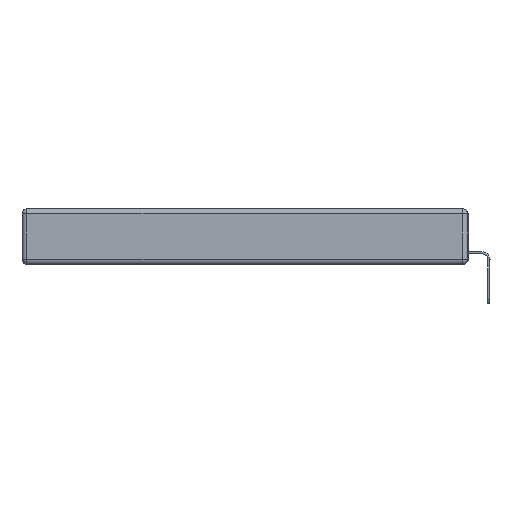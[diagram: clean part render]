
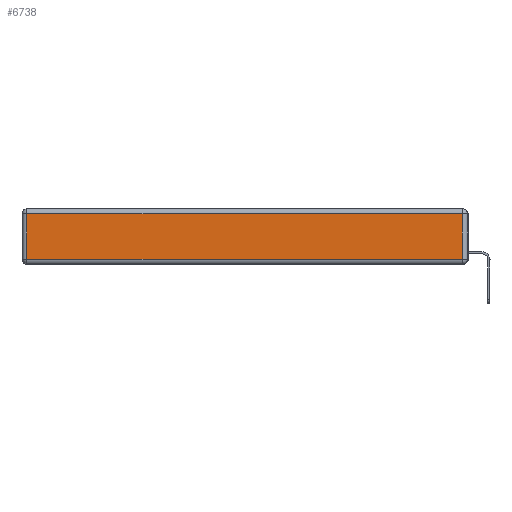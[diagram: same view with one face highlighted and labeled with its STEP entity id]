
A CAD part, left-side view. The second image highlights one B-rep face of the part: STEP entity #6738.
In plain terms, the highlighted planar face has unit normal (-1, 0, 0).
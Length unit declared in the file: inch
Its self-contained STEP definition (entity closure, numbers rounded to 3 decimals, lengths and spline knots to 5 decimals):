
#150 = CARTESIAN_POINT ( 'NONE',  ( 0., 0.03, -0.343 ) ) ;
#825 = ORIENTED_EDGE ( 'NONE', *, *, #14032, .T. ) ;
#1256 = EDGE_LOOP ( 'NONE', ( #825, #8724, #1571, #6125 ) ) ;
#1292 = EDGE_CURVE ( 'NONE', #6046, #7868, #12405, .T. ) ;
#1571 = ORIENTED_EDGE ( 'NONE', *, *, #3129, .T. ) ;
#1878 = DIRECTION ( 'NONE',  ( 0., 0., -1. ) ) ;
#2575 = LINE ( 'NONE', #16299, #7456 ) ;
#3129 = EDGE_CURVE ( 'NONE', #15736, #6046, #2575, .T. ) ;
#3738 = VECTOR ( 'NONE', #7535, 39.37008 ) ;
#3893 = PLANE ( 'NONE',  #14720 ) ;
#4671 = VECTOR ( 'NONE', #1878, 39.37008 ) ;
#5703 = VERTEX_POINT ( 'NONE', #11118 ) ;
#6046 = VERTEX_POINT ( 'NONE', #9360 ) ;
#6125 = ORIENTED_EDGE ( 'NONE', *, *, #1292, .T. ) ;
#6738 = ADVANCED_FACE ( 'NONE', ( #8575 ), #3893, .T. ) ;
#7260 = LINE ( 'NONE', #150, #15590 ) ;
#7456 = VECTOR ( 'NONE', #16352, 39.37008 ) ;
#7535 = DIRECTION ( 'NONE',  ( 0., -1., 0. ) ) ;
#7868 = VERTEX_POINT ( 'NONE', #11662 ) ;
#7915 = DIRECTION ( 'NONE',  ( -1., 0., 0. ) ) ;
#8575 = FACE_OUTER_BOUND ( 'NONE', #1256, .T. ) ;
#8724 = ORIENTED_EDGE ( 'NONE', *, *, #11621, .T. ) ;
#9360 = CARTESIAN_POINT ( 'NONE',  ( 0., 2.72, -0.03 ) ) ;
#10305 = DIRECTION ( 'NONE',  ( 0., 0., 1. ) ) ;
#11118 = CARTESIAN_POINT ( 'NONE',  ( 0., 0.03, -0.313 ) ) ;
#11132 = CARTESIAN_POINT ( 'NONE',  ( 0., 0.03, -0.03 ) ) ;
#11621 = EDGE_CURVE ( 'NONE', #5703, #15736, #7260, .T. ) ;
#11662 = CARTESIAN_POINT ( 'NONE',  ( 0., 2.72, -0.313 ) ) ;
#12405 = LINE ( 'NONE', #16256, #4671 ) ;
#12917 = LINE ( 'NONE', #15340, #3738 ) ;
#14032 = EDGE_CURVE ( 'NONE', #7868, #5703, #12917, .T. ) ;
#14720 = AXIS2_PLACEMENT_3D ( 'NONE', #16853, #7915, #10305 ) ;
#15340 = CARTESIAN_POINT ( 'NONE',  ( 0., 0., -0.313 ) ) ;
#15590 = VECTOR ( 'NONE', #15679, 39.37008 ) ;
#15679 = DIRECTION ( 'NONE',  ( 0., 0., 1. ) ) ;
#15736 = VERTEX_POINT ( 'NONE', #11132 ) ;
#16256 = CARTESIAN_POINT ( 'NONE',  ( 0., 2.72, -0.343 ) ) ;
#16299 = CARTESIAN_POINT ( 'NONE',  ( 0., 2.75, -0.03 ) ) ;
#16352 = DIRECTION ( 'NONE',  ( 0., 1., 0. ) ) ;
#16853 = CARTESIAN_POINT ( 'NONE',  ( 0., 0., -0.343 ) ) ;
